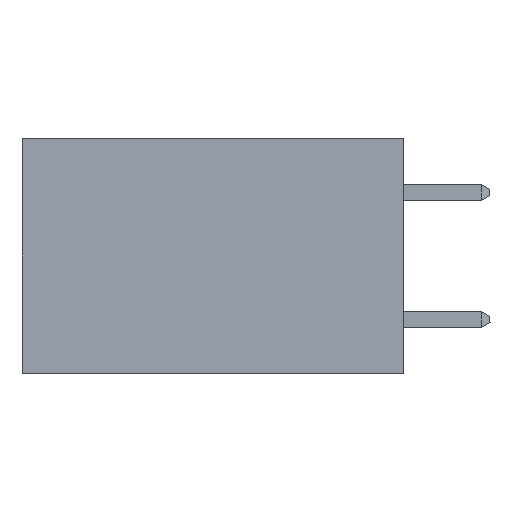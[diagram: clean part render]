
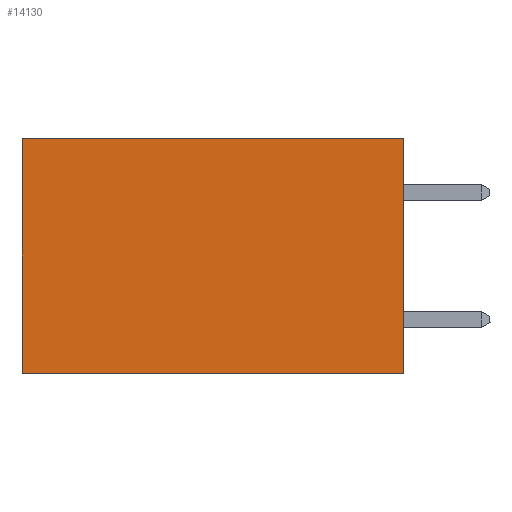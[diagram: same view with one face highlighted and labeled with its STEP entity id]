
A CAD part, left-side view. The second image highlights one B-rep face of the part: STEP entity #14130.
In plain terms, the highlighted planar face has unit normal (-1, 0, 0).
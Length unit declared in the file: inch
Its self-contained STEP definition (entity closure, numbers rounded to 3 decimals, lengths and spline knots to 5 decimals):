
#257 = LINE ( 'NONE', #10691, #4435 ) ;
#1676 = CARTESIAN_POINT ( 'NONE',  ( 0.2875, 0., -0.37 ) ) ;
#2391 = CARTESIAN_POINT ( 'NONE',  ( 0.2875, 0.6, -0.37 ) ) ;
#3658 = LINE ( 'NONE', #17891, #31315 ) ;
#4412 = EDGE_CURVE ( 'NONE', #16557, #13902, #3658, .T. ) ;
#4435 = VECTOR ( 'NONE', #10348, 39.37008 ) ;
#5097 = DIRECTION ( 'NONE',  ( 0., 1., 0. ) ) ;
#6949 = CARTESIAN_POINT ( 'NONE',  ( 0.2875, 0., 0. ) ) ;
#7767 = DIRECTION ( 'NONE',  ( 0., 0., -1. ) ) ;
#8777 = EDGE_LOOP ( 'NONE', ( #18981, #26699, #26681, #14932 ) ) ;
#10348 = DIRECTION ( 'NONE',  ( 0., 0., -1. ) ) ;
#10691 = CARTESIAN_POINT ( 'NONE',  ( 0.2875, 0., 0. ) ) ;
#12710 = VERTEX_POINT ( 'NONE', #27067 ) ;
#12851 = EDGE_CURVE ( 'NONE', #13902, #21607, #13125, .T. ) ;
#13125 = LINE ( 'NONE', #29079, #23623 ) ;
#13902 = VERTEX_POINT ( 'NONE', #28649 ) ;
#14130 = ADVANCED_FACE ( 'NONE', ( #20597 ), #20015, .F. ) ;
#14349 = VECTOR ( 'NONE', #5097, 39.37008 ) ;
#14932 = ORIENTED_EDGE ( 'NONE', *, *, #4412, .T. ) ;
#16557 = VERTEX_POINT ( 'NONE', #6949 ) ;
#17891 = CARTESIAN_POINT ( 'NONE',  ( 0.2875, 0., 0. ) ) ;
#18981 = ORIENTED_EDGE ( 'NONE', *, *, #12851, .T. ) ;
#19806 = DIRECTION ( 'NONE',  ( 1., 0., 0. ) ) ;
#20015 = PLANE ( 'NONE',  #22865 ) ;
#20597 = FACE_OUTER_BOUND ( 'NONE', #8777, .T. ) ;
#21607 = VERTEX_POINT ( 'NONE', #2391 ) ;
#22865 = AXIS2_PLACEMENT_3D ( 'NONE', #25514, #19806, #30471 ) ;
#23025 = EDGE_CURVE ( 'NONE', #12710, #21607, #28590, .T. ) ;
#23623 = VECTOR ( 'NONE', #7767, 39.37008 ) ;
#25514 = CARTESIAN_POINT ( 'NONE',  ( 0.2875, 0., 0. ) ) ;
#26681 = ORIENTED_EDGE ( 'NONE', *, *, #27998, .F. ) ;
#26699 = ORIENTED_EDGE ( 'NONE', *, *, #23025, .F. ) ;
#27067 = CARTESIAN_POINT ( 'NONE',  ( 0.2875, 0., -0.37 ) ) ;
#27998 = EDGE_CURVE ( 'NONE', #16557, #12710, #257, .T. ) ;
#28590 = LINE ( 'NONE', #1676, #14349 ) ;
#28649 = CARTESIAN_POINT ( 'NONE',  ( 0.2875, 0.6, 0. ) ) ;
#29079 = CARTESIAN_POINT ( 'NONE',  ( 0.2875, 0.6, 0. ) ) ;
#30471 = DIRECTION ( 'NONE',  ( 0., 0., -1. ) ) ;
#31315 = VECTOR ( 'NONE', #33740, 39.37008 ) ;
#33740 = DIRECTION ( 'NONE',  ( 0., 1., 0. ) ) ;
